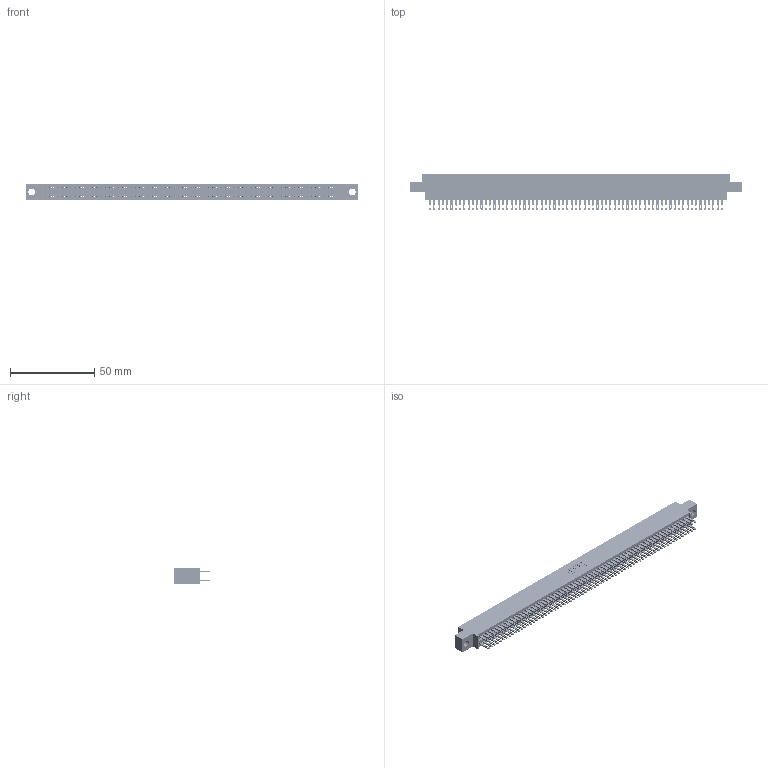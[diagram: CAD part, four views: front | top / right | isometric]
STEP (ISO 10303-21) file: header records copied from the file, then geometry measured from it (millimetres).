
FILE_DESCRIPTION (( 'STEP AP203' ), '1' );
FILE_NAME ('345-138-500-804.STEP', '2021-05-25T23:44:50', ( '' ), ( '' ), 'SwSTEP 2.0', 'SolidWorks 2020', '' );
FILE_SCHEMA (( 'CONFIG_CONTROL_DESIGN' ));
Length unit declared in the file: inch
Products named in the file (3): 345-292-001_345-293-100; 345-138-500-804; 345 Part_0.170 Offset - 0.156 Dia-TI
Assembly tree (139 placements, depth 2):
  345-138-500-804
    345 Part_0.170 Offset - 0.156 Dia-TI
    345-292-001_345-293-100  x138
Bounding box: 196.47 x 21.51 x 9.4 mm (x, y, z)
Volume: 19538.2 mm3; surface area: 30806.2 mm2
Topology: 139 solids, 139 shells, 6492 faces, 19847 edges, 13230 vertices
Faces by surface type: plane 3824, cylinder 2668
Entity records: 50985 total; most frequent: CARTESIAN_POINT 8526, ORIENTED_EDGE 8458, DIRECTION 7485, EDGE_CURVE 4229, VECTOR 3817, LINE 3817, VERTEX_POINT 2818, AXIS2_PLACEMENT_3D 1834
